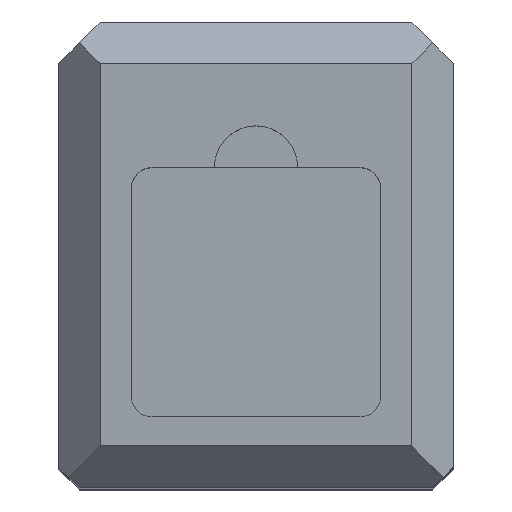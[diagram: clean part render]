
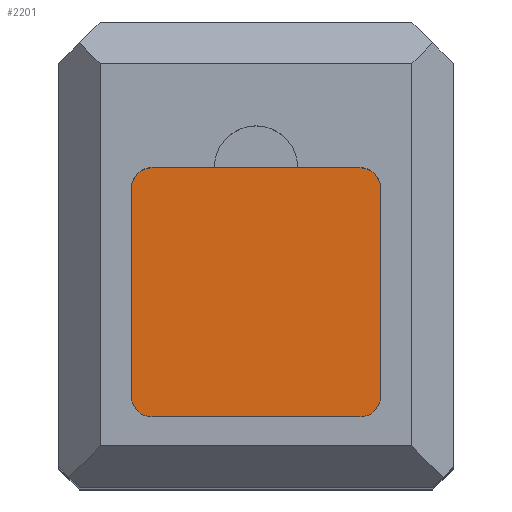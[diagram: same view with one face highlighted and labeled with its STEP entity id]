
A CAD part, top view. The second image highlights one B-rep face of the part: STEP entity #2201.
In plain terms, the highlighted planar face has unit normal (0, 0, 1).
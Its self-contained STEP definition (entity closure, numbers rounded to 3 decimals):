
#141=CARTESIAN_POINT('',(-5.,6.,-11.));
#142=VERTEX_POINT('',#141);
#149=CARTESIAN_POINT('',(5.,6.,-11.));
#150=VERTEX_POINT('',#149);
#151=CARTESIAN_POINT('',(-5.,6.,-11.));
#152=DIRECTION('',(1.0,0.0,0.0));
#153=VECTOR('',#152,10.);
#154=LINE('',#151,#153);
#155=EDGE_CURVE('',#142,#150,#154,.T.);
#2101=CARTESIAN_POINT('',(-6.,5.0,-11.));
#2102=VERTEX_POINT('',#2101);
#2103=CARTESIAN_POINT('',(-5.,5.,-11.));
#2104=DIRECTION('',(0.0,0.0,1.0));
#2105=DIRECTION('',(-0.707,0.707,0.0));
#2106=AXIS2_PLACEMENT_3D('',#2103,#2104,#2105);
#2107=CIRCLE('',#2106,1.0);
#2108=EDGE_CURVE('',#142,#2102,#2107,.T.);
#2126=CARTESIAN_POINT('',(-6.,-5.,-11.));
#2127=VERTEX_POINT('',#2126);
#2128=CARTESIAN_POINT('',(-5.,-6.,-11.));
#2129=VERTEX_POINT('',#2128);
#2130=CARTESIAN_POINT('',(-5.,-5.,-11.));
#2131=DIRECTION('',(0.0,0.0,1.0));
#2132=DIRECTION('',(-0.707,-0.707,0.0));
#2133=AXIS2_PLACEMENT_3D('',#2130,#2131,#2132);
#2134=CIRCLE('',#2133,1.0);
#2135=EDGE_CURVE('',#2127,#2129,#2134,.T.);
#2153=CARTESIAN_POINT('',(0.0,6.,-11.));
#2154=DIRECTION('',(0.0,0.0,-1.0));
#2155=DIRECTION('',(-1.0,0.0,0.0));
#2156=AXIS2_PLACEMENT_3D('',#2153,#2154,#2155);
#2157=PLANE('',#2156);
#2158=ORIENTED_EDGE('',*,*,#2108,.T.);
#2159=CARTESIAN_POINT('',(-6.,-5.,-11.));
#2160=DIRECTION('',(0.0,1.0,0.0));
#2161=VECTOR('',#2160,10.0);
#2162=LINE('',#2159,#2161);
#2163=EDGE_CURVE('',#2127,#2102,#2162,.T.);
#2164=ORIENTED_EDGE('',*,*,#2163,.F.);
#2165=ORIENTED_EDGE('',*,*,#2135,.T.);
#2166=CARTESIAN_POINT('',(5.,-6.,-11.));
#2167=VERTEX_POINT('',#2166);
#2168=CARTESIAN_POINT('',(-5.,-6.,-11.));
#2169=DIRECTION('',(1.0,0.0,0.0));
#2170=VECTOR('',#2169,10.);
#2171=LINE('',#2168,#2170);
#2172=EDGE_CURVE('',#2129,#2167,#2171,.T.);
#2173=ORIENTED_EDGE('',*,*,#2172,.T.);
#2174=CARTESIAN_POINT('',(6.,-5.,-11.));
#2175=VERTEX_POINT('',#2174);
#2176=CARTESIAN_POINT('',(5.,-5.,-11.));
#2177=DIRECTION('',(0.0,0.0,1.0));
#2178=DIRECTION('',(0.707,-0.707,0.0));
#2179=AXIS2_PLACEMENT_3D('',#2176,#2177,#2178);
#2180=CIRCLE('',#2179,1.0);
#2181=EDGE_CURVE('',#2167,#2175,#2180,.T.);
#2182=ORIENTED_EDGE('',*,*,#2181,.T.);
#2183=CARTESIAN_POINT('',(6.,5.0,-11.));
#2184=VERTEX_POINT('',#2183);
#2185=CARTESIAN_POINT('',(6.,5.,-11.));
#2186=DIRECTION('',(0.0,-1.0,0.0));
#2187=VECTOR('',#2186,10.0);
#2188=LINE('',#2185,#2187);
#2189=EDGE_CURVE('',#2184,#2175,#2188,.T.);
#2190=ORIENTED_EDGE('',*,*,#2189,.F.);
#2191=CARTESIAN_POINT('',(5.,5.,-11.));
#2192=DIRECTION('',(0.0,0.0,1.0));
#2193=DIRECTION('',(0.707,0.707,0.0));
#2194=AXIS2_PLACEMENT_3D('',#2191,#2192,#2193);
#2195=CIRCLE('',#2194,1.0);
#2196=EDGE_CURVE('',#2184,#150,#2195,.T.);
#2197=ORIENTED_EDGE('',*,*,#2196,.T.);
#2198=ORIENTED_EDGE('',*,*,#155,.F.);
#2199=EDGE_LOOP('',(#2158,#2164,#2165,#2173,#2182,#2190,#2197,#2198));
#2200=FACE_OUTER_BOUND('',#2199,.T.);
#2201=ADVANCED_FACE('',(#2200),#2157,.F.);
